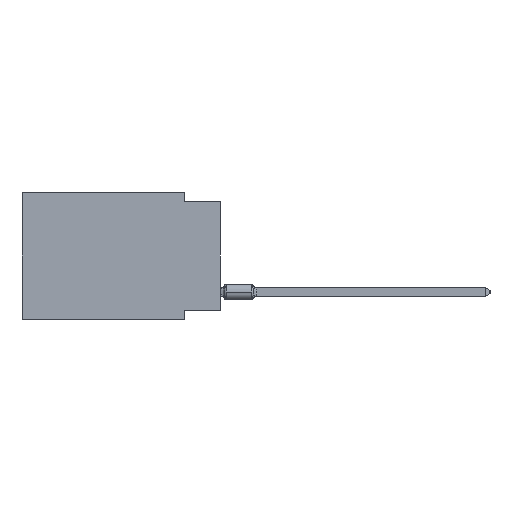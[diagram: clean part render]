
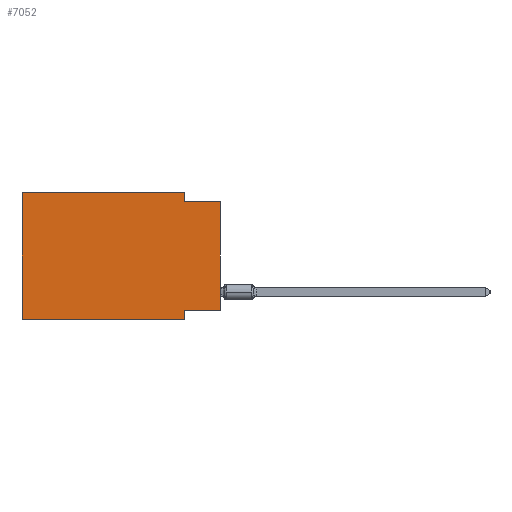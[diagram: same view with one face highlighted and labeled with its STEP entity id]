
A CAD part, left-side view. The second image highlights one B-rep face of the part: STEP entity #7052.
In plain terms, the highlighted planar face has unit normal (-1, 0, 0).
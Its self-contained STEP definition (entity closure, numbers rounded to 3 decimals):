
#479 = ORIENTED_EDGE ( 'NONE', *, *, #663, .F. ) ;
#663 = EDGE_CURVE ( 'NONE', #15802, #10740, #7296, .T. ) ;
#973 = VECTOR ( 'NONE', #21754, 1000. ) ;
#1027 = DIRECTION ( 'NONE',  ( 0., -1., 0. ) ) ;
#1098 = VECTOR ( 'NONE', #3581, 1000. ) ;
#1828 = CARTESIAN_POINT ( 'NONE',  ( 0., 0., 0. ) ) ;
#1960 = CARTESIAN_POINT ( 'NONE',  ( 0., 13.97, 0. ) ) ;
#2033 = EDGE_CURVE ( 'NONE', #23204, #3075, #11968, .T. ) ;
#2205 = VERTEX_POINT ( 'NONE', #17315 ) ;
#2379 = ORIENTED_EDGE ( 'NONE', *, *, #17612, .F. ) ;
#2902 = EDGE_CURVE ( 'NONE', #22465, #9764, #3587, .T. ) ;
#3075 = VERTEX_POINT ( 'NONE', #10743 ) ;
#3581 = DIRECTION ( 'NONE',  ( 0., 0., -1. ) ) ;
#3587 = LINE ( 'NONE', #15850, #23919 ) ;
#3661 = EDGE_CURVE ( 'NONE', #23204, #10740, #13697, .T. ) ;
#3819 = EDGE_CURVE ( 'NONE', #11600, #2205, #24107, .T. ) ;
#4189 = VECTOR ( 'NONE', #24034, 1000. ) ;
#4235 = EDGE_CURVE ( 'NONE', #3075, #9764, #19248, .T. ) ;
#4474 = LINE ( 'NONE', #8136, #4189 ) ;
#4968 = ORIENTED_EDGE ( 'NONE', *, *, #3661, .T. ) ;
#5408 = DIRECTION ( 'NONE',  ( 0., 0., -1. ) ) ;
#6064 = VECTOR ( 'NONE', #18105, 1000. ) ;
#7052 = ADVANCED_FACE ( 'NONE', ( #25233 ), #11665, .F. ) ;
#7159 = EDGE_LOOP ( 'NONE', ( #4968, #479, #2379, #18135, #19610, #13474, #16503, #23540 ) ) ;
#7296 = LINE ( 'NONE', #10937, #24772 ) ;
#7322 = DIRECTION ( 'NONE',  ( 0., 0., 1. ) ) ;
#8136 = CARTESIAN_POINT ( 'NONE',  ( 0., 13.97, 0. ) ) ;
#9764 = VERTEX_POINT ( 'NONE', #16309 ) ;
#10680 = LINE ( 'NONE', #19136, #23153 ) ;
#10740 = VERTEX_POINT ( 'NONE', #15870 ) ;
#10743 = CARTESIAN_POINT ( 'NONE',  ( 0., 2.54, -8.255 ) ) ;
#10937 = CARTESIAN_POINT ( 'NONE',  ( 0., 0., -0.635 ) ) ;
#11593 = CARTESIAN_POINT ( 'NONE',  ( 0., 0., -8.255 ) ) ;
#11600 = VERTEX_POINT ( 'NONE', #24377 ) ;
#11665 = PLANE ( 'NONE',  #21996 ) ;
#11968 = LINE ( 'NONE', #11593, #973 ) ;
#12252 = EDGE_CURVE ( 'NONE', #22465, #11600, #4474, .T. ) ;
#12497 = CARTESIAN_POINT ( 'NONE',  ( 0., 0., -8.255 ) ) ;
#13339 = CARTESIAN_POINT ( 'NONE',  ( 0., 13.97, -8.89 ) ) ;
#13474 = ORIENTED_EDGE ( 'NONE', *, *, #2902, .T. ) ;
#13697 = LINE ( 'NONE', #1828, #23544 ) ;
#13748 = DIRECTION ( 'NONE',  ( 1., 0., 0. ) ) ;
#15802 = VERTEX_POINT ( 'NONE', #17229 ) ;
#15850 = CARTESIAN_POINT ( 'NONE',  ( 0., 13.97, -8.89 ) ) ;
#15870 = CARTESIAN_POINT ( 'NONE',  ( 0., 0., -0.635 ) ) ;
#16309 = CARTESIAN_POINT ( 'NONE',  ( 0., 2.54, -8.89 ) ) ;
#16503 = ORIENTED_EDGE ( 'NONE', *, *, #4235, .F. ) ;
#17229 = CARTESIAN_POINT ( 'NONE',  ( 0., 2.54, -0.635 ) ) ;
#17315 = CARTESIAN_POINT ( 'NONE',  ( 0., 2.54, 0. ) ) ;
#17612 = EDGE_CURVE ( 'NONE', #2205, #15802, #10680, .T. ) ;
#18105 = DIRECTION ( 'NONE',  ( 0., -1., 0. ) ) ;
#18135 = ORIENTED_EDGE ( 'NONE', *, *, #3819, .F. ) ;
#19120 = CARTESIAN_POINT ( 'NONE',  ( 0., 2.54, -8.89 ) ) ;
#19136 = CARTESIAN_POINT ( 'NONE',  ( 0., 2.54, 0. ) ) ;
#19248 = LINE ( 'NONE', #19120, #1098 ) ;
#19610 = ORIENTED_EDGE ( 'NONE', *, *, #12252, .F. ) ;
#19640 = CARTESIAN_POINT ( 'NONE',  ( 0., 13.97, 0. ) ) ;
#20601 = DIRECTION ( 'NONE',  ( 0., 0., -1. ) ) ;
#21754 = DIRECTION ( 'NONE',  ( 0., 1., 0. ) ) ;
#21996 = AXIS2_PLACEMENT_3D ( 'NONE', #19640, #13748, #5408 ) ;
#22465 = VERTEX_POINT ( 'NONE', #13339 ) ;
#23153 = VECTOR ( 'NONE', #20601, 1000. ) ;
#23204 = VERTEX_POINT ( 'NONE', #12497 ) ;
#23540 = ORIENTED_EDGE ( 'NONE', *, *, #2033, .F. ) ;
#23544 = VECTOR ( 'NONE', #7322, 1000. ) ;
#23794 = DIRECTION ( 'NONE',  ( 0., -1., 0. ) ) ;
#23919 = VECTOR ( 'NONE', #23794, 1000. ) ;
#24034 = DIRECTION ( 'NONE',  ( 0., 0., 1. ) ) ;
#24107 = LINE ( 'NONE', #1960, #6064 ) ;
#24377 = CARTESIAN_POINT ( 'NONE',  ( 0., 13.97, 0. ) ) ;
#24772 = VECTOR ( 'NONE', #1027, 1000. ) ;
#25233 = FACE_OUTER_BOUND ( 'NONE', #7159, .T. ) ;
